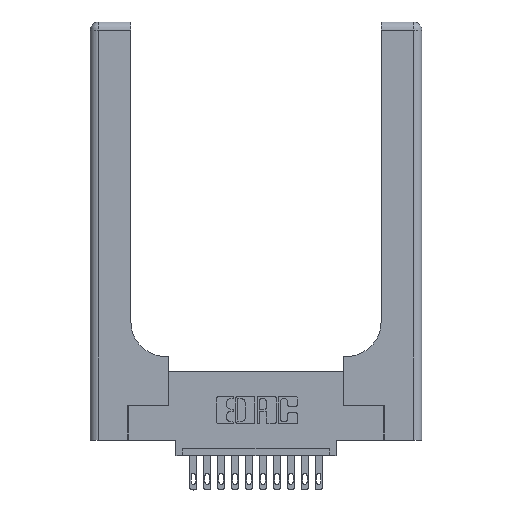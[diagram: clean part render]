
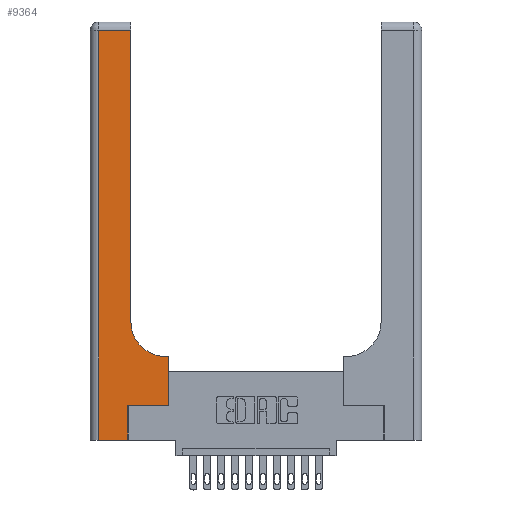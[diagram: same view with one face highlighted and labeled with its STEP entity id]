
A CAD part, top view. The second image highlights one B-rep face of the part: STEP entity #9364.
In plain terms, the highlighted planar face has unit normal (0, 0, 1).
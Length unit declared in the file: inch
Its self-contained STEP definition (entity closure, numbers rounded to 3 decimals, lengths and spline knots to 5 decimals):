
#425 = DIRECTION ( 'NONE',  ( -1., 0., 0. ) ) ;
#466 = VERTEX_POINT ( 'NONE', #10641 ) ;
#467 = VECTOR ( 'NONE', #12906, 39.37008 ) ;
#586 = VECTOR ( 'NONE', #10319, 39.37008 ) ;
#805 = LINE ( 'NONE', #6835, #5766 ) ;
#845 = AXIS2_PLACEMENT_3D ( 'NONE', #8670, #4679, #13947 ) ;
#885 = CARTESIAN_POINT ( 'NONE',  ( 0.2915, 2.94, 0.37 ) ) ;
#1046 = VECTOR ( 'NONE', #425, 39.37008 ) ;
#1581 = DIRECTION ( 'NONE',  ( 0., 1., 0. ) ) ;
#1719 = VECTOR ( 'NONE', #12930, 39.37008 ) ;
#1725 = ORIENTED_EDGE ( 'NONE', *, *, #11605, .T. ) ;
#2333 = VERTEX_POINT ( 'NONE', #5325 ) ;
#2663 = CARTESIAN_POINT ( 'NONE',  ( 0.5415, 0.6, 0.37 ) ) ;
#2778 = EDGE_CURVE ( 'NONE', #6203, #11509, #16958, .T. ) ;
#3602 = CARTESIAN_POINT ( 'NONE',  ( 0., 0., 0.37 ) ) ;
#3610 = CARTESIAN_POINT ( 'NONE',  ( 0.06, 3., 0.37 ) ) ;
#3624 = ORIENTED_EDGE ( 'NONE', *, *, #4555, .T. ) ;
#4116 = LINE ( 'NONE', #3602, #586 ) ;
#4190 = PLANE ( 'NONE',  #6722 ) ;
#4555 = EDGE_CURVE ( 'NONE', #14911, #10241, #8868, .T. ) ;
#4679 = DIRECTION ( 'NONE',  ( 0., 0., -1. ) ) ;
#4813 = LINE ( 'NONE', #14206, #467 ) ;
#4834 = CARTESIAN_POINT ( 'NONE',  ( 0.269, 0., 0.37 ) ) ;
#4907 = ORIENTED_EDGE ( 'NONE', *, *, #14794, .T. ) ;
#5325 = CARTESIAN_POINT ( 'NONE',  ( 0.2915, 0.85, 0.37 ) ) ;
#5341 = FACE_OUTER_BOUND ( 'NONE', #9543, .T. ) ;
#5579 = CARTESIAN_POINT ( 'NONE',  ( 0.06, 2.94, 0.37 ) ) ;
#5766 = VECTOR ( 'NONE', #1581, 39.37008 ) ;
#5959 = ORIENTED_EDGE ( 'NONE', *, *, #6884, .T. ) ;
#6203 = VERTEX_POINT ( 'NONE', #16384 ) ;
#6343 = LINE ( 'NONE', #3610, #7744 ) ;
#6722 = AXIS2_PLACEMENT_3D ( 'NONE', #13386, #12231, #13570 ) ;
#6833 = EDGE_CURVE ( 'NONE', #2333, #11215, #4813, .T. ) ;
#6835 = CARTESIAN_POINT ( 'NONE',  ( 0.5585, 0.25, 0.37 ) ) ;
#6866 = CARTESIAN_POINT ( 'NONE',  ( 0.2915, 0.6, 0.37 ) ) ;
#6884 = EDGE_CURVE ( 'NONE', #10241, #2333, #7852, .T. ) ;
#7744 = VECTOR ( 'NONE', #11444, 39.37008 ) ;
#7852 = CIRCLE ( 'NONE', #845, 0.25 ) ;
#8131 = ORIENTED_EDGE ( 'NONE', *, *, #10361, .T. ) ;
#8276 = DIRECTION ( 'NONE',  ( 1., 0., 0. ) ) ;
#8670 = CARTESIAN_POINT ( 'NONE',  ( 0.5415, 0.85, 0.37 ) ) ;
#8868 = LINE ( 'NONE', #6866, #1046 ) ;
#9364 = ADVANCED_FACE ( 'NONE', ( #5341 ), #4190, .F. ) ;
#9543 = EDGE_LOOP ( 'NONE', ( #15156, #4907, #10729, #1725, #10657, #8131, #13665, #3624, #5959 ) ) ;
#10241 = VERTEX_POINT ( 'NONE', #2663 ) ;
#10319 = DIRECTION ( 'NONE',  ( 1., 0., 0. ) ) ;
#10344 = EDGE_CURVE ( 'NONE', #466, #14911, #805, .T. ) ;
#10361 = EDGE_CURVE ( 'NONE', #11509, #466, #14441, .T. ) ;
#10641 = CARTESIAN_POINT ( 'NONE',  ( 0.5585, 0.25, 0.37 ) ) ;
#10657 = ORIENTED_EDGE ( 'NONE', *, *, #2778, .T. ) ;
#10729 = ORIENTED_EDGE ( 'NONE', *, *, #11055, .T. ) ;
#11055 = EDGE_CURVE ( 'NONE', #16901, #14235, #6343, .T. ) ;
#11123 = VECTOR ( 'NONE', #14922, 39.37008 ) ;
#11215 = VERTEX_POINT ( 'NONE', #885 ) ;
#11444 = DIRECTION ( 'NONE',  ( 0., -1., 0. ) ) ;
#11509 = VERTEX_POINT ( 'NONE', #12504 ) ;
#11605 = EDGE_CURVE ( 'NONE', #14235, #6203, #4116, .T. ) ;
#12231 = DIRECTION ( 'NONE',  ( 0., 0., -1. ) ) ;
#12504 = CARTESIAN_POINT ( 'NONE',  ( 0.269, 0.25, 0.37 ) ) ;
#12906 = DIRECTION ( 'NONE',  ( 0., 1., 0. ) ) ;
#12930 = DIRECTION ( 'NONE',  ( 0., 1., 0. ) ) ;
#13386 = CARTESIAN_POINT ( 'NONE',  ( 0., 3., 0.37 ) ) ;
#13570 = DIRECTION ( 'NONE',  ( -1., 0., 0. ) ) ;
#13665 = ORIENTED_EDGE ( 'NONE', *, *, #10344, .T. ) ;
#13947 = DIRECTION ( 'NONE',  ( 1., 0., 0. ) ) ;
#14206 = CARTESIAN_POINT ( 'NONE',  ( 0.2915, 3., 0.37 ) ) ;
#14235 = VERTEX_POINT ( 'NONE', #15903 ) ;
#14441 = LINE ( 'NONE', #16173, #15050 ) ;
#14794 = EDGE_CURVE ( 'NONE', #11215, #16901, #15051, .T. ) ;
#14911 = VERTEX_POINT ( 'NONE', #16549 ) ;
#14922 = DIRECTION ( 'NONE',  ( -1., 0., 0. ) ) ;
#15031 = CARTESIAN_POINT ( 'NONE',  ( 0., 2.94, 0.37 ) ) ;
#15050 = VECTOR ( 'NONE', #8276, 39.37008 ) ;
#15051 = LINE ( 'NONE', #15031, #11123 ) ;
#15156 = ORIENTED_EDGE ( 'NONE', *, *, #6833, .T. ) ;
#15903 = CARTESIAN_POINT ( 'NONE',  ( 0.06, 0., 0.37 ) ) ;
#16173 = CARTESIAN_POINT ( 'NONE',  ( 0.269, 0.25, 0.37 ) ) ;
#16384 = CARTESIAN_POINT ( 'NONE',  ( 0.269, 0., 0.37 ) ) ;
#16549 = CARTESIAN_POINT ( 'NONE',  ( 0.5585, 0.6, 0.37 ) ) ;
#16901 = VERTEX_POINT ( 'NONE', #5579 ) ;
#16958 = LINE ( 'NONE', #4834, #1719 ) ;
